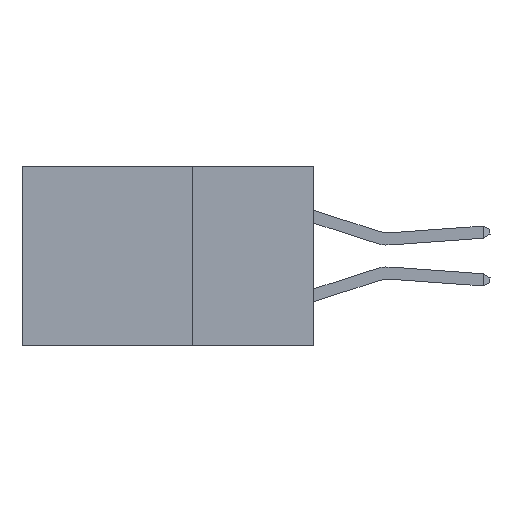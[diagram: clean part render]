
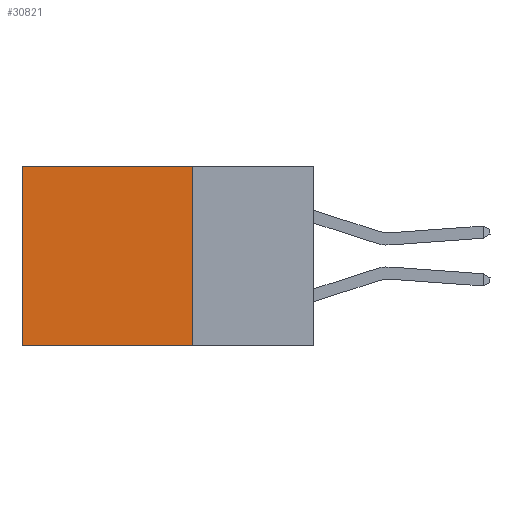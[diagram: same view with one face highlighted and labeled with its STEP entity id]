
A CAD part, left-side view. The second image highlights one B-rep face of the part: STEP entity #30821.
In plain terms, the highlighted planar face has unit normal (-1, 0, 0).
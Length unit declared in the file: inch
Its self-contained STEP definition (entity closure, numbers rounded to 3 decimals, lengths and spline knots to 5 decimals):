
#1513 = CARTESIAN_POINT ( 'NONE',  ( 0.2875, 0.25, 0. ) ) ;
#1672 = DIRECTION ( 'NONE',  ( 0., 0., -1. ) ) ;
#4097 = VECTOR ( 'NONE', #37475, 39.37008 ) ;
#5778 = LINE ( 'NONE', #38971, #21044 ) ;
#8029 = CARTESIAN_POINT ( 'NONE',  ( 0.2875, 0.6, 0. ) ) ;
#10562 = ORIENTED_EDGE ( 'NONE', *, *, #22992, .F. ) ;
#11751 = VERTEX_POINT ( 'NONE', #30136 ) ;
#13250 = ORIENTED_EDGE ( 'NONE', *, *, #15716, .T. ) ;
#13507 = ORIENTED_EDGE ( 'NONE', *, *, #37453, .T. ) ;
#13985 = CARTESIAN_POINT ( 'NONE',  ( 0.2875, 0.25, -0.37 ) ) ;
#15357 = AXIS2_PLACEMENT_3D ( 'NONE', #40338, #29750, #16700 ) ;
#15716 = EDGE_CURVE ( 'NONE', #11751, #43032, #5778, .T. ) ;
#16140 = LINE ( 'NONE', #8029, #21380 ) ;
#16700 = DIRECTION ( 'NONE',  ( 0., 0., -1. ) ) ;
#18305 = DIRECTION ( 'NONE',  ( 0., 1., 0. ) ) ;
#19231 = FACE_OUTER_BOUND ( 'NONE', #27494, .T. ) ;
#21044 = VECTOR ( 'NONE', #18305, 39.37008 ) ;
#21346 = VECTOR ( 'NONE', #41178, 39.37008 ) ;
#21380 = VECTOR ( 'NONE', #1672, 39.37008 ) ;
#22992 = EDGE_CURVE ( 'NONE', #11751, #27980, #42320, .T. ) ;
#24792 = CARTESIAN_POINT ( 'NONE',  ( 0.2875, 0.6, 0. ) ) ;
#26376 = PLANE ( 'NONE',  #15357 ) ;
#26986 = CARTESIAN_POINT ( 'NONE',  ( 0.2875, 0.6, -0.37 ) ) ;
#27494 = EDGE_LOOP ( 'NONE', ( #13507, #41146, #10562, #13250 ) ) ;
#27980 = VERTEX_POINT ( 'NONE', #36190 ) ;
#29750 = DIRECTION ( 'NONE',  ( 1., 0., 0. ) ) ;
#30136 = CARTESIAN_POINT ( 'NONE',  ( 0.2875, 0.25, 0. ) ) ;
#30821 = ADVANCED_FACE ( 'NONE', ( #19231 ), #26376, .F. ) ;
#33096 = VERTEX_POINT ( 'NONE', #26986 ) ;
#36190 = CARTESIAN_POINT ( 'NONE',  ( 0.2875, 0.25, -0.37 ) ) ;
#37453 = EDGE_CURVE ( 'NONE', #43032, #33096, #16140, .T. ) ;
#37475 = DIRECTION ( 'NONE',  ( 0., 1., 0. ) ) ;
#38486 = EDGE_CURVE ( 'NONE', #27980, #33096, #43434, .T. ) ;
#38971 = CARTESIAN_POINT ( 'NONE',  ( 0.2875, 0.25, 0. ) ) ;
#40338 = CARTESIAN_POINT ( 'NONE',  ( 0.2875, 0.25, 0. ) ) ;
#41146 = ORIENTED_EDGE ( 'NONE', *, *, #38486, .F. ) ;
#41178 = DIRECTION ( 'NONE',  ( 0., 0., -1. ) ) ;
#42320 = LINE ( 'NONE', #1513, #21346 ) ;
#43032 = VERTEX_POINT ( 'NONE', #24792 ) ;
#43434 = LINE ( 'NONE', #13985, #4097 ) ;
